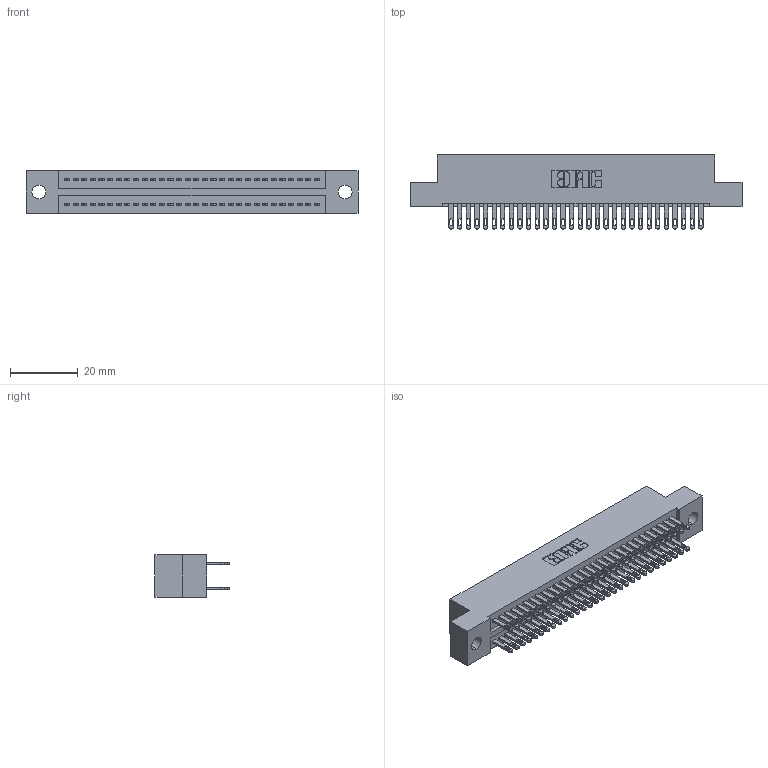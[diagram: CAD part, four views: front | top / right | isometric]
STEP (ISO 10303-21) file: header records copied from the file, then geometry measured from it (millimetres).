
FILE_DESCRIPTION (( 'STEP AP203' ), '1' );
FILE_NAME ('325-060-500-209.STEP', '2020-02-25T02:27:38', ( '' ), ( '' ), 'SwSTEP 2.0', 'SolidWorks 2016', '' );
FILE_SCHEMA (( 'CONFIG_CONTROL_DESIGN' ));
Length unit declared in the file: inch
Products named in the file (3): 325-060-500-209; 325-292-001_325-293-100; 325 Part_.160 TH
Assembly tree (61 placements, depth 2):
  325-060-500-209
    325 Part_.160 TH
    325-292-001_325-293-100  x60
Bounding box: 97.92 x 21.84 x 12.45 mm (x, y, z)
Volume: 12485.5 mm3; surface area: 15375.3 mm2
Topology: 61 solids, 61 shells, 2994 faces, 9131 edges, 6086 vertices
Faces by surface type: plane 1870, cylinder 1124
Entity records: 20785 total; most frequent: CARTESIAN_POINT 3458, ORIENTED_EDGE 3394, DIRECTION 2977, EDGE_CURVE 1697, VECTOR 1565, LINE 1565, VERTEX_POINT 1130, AXIS2_PLACEMENT_3D 706
